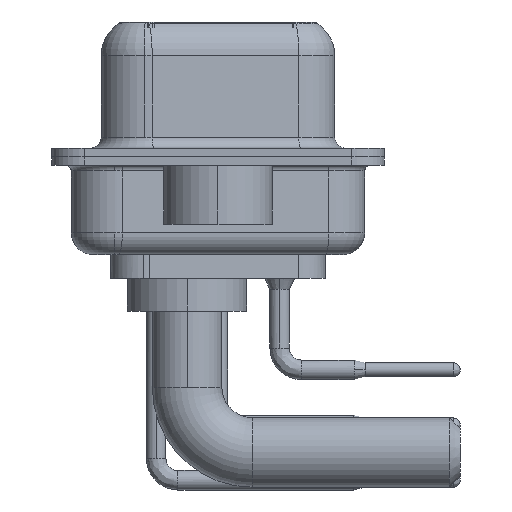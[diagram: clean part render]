
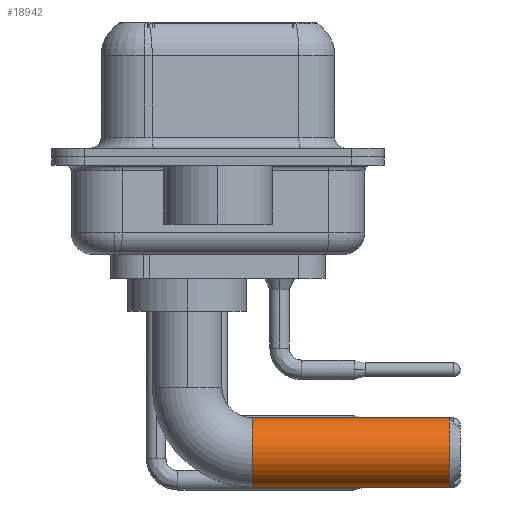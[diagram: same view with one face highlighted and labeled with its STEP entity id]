
A CAD part, left-side view. The second image highlights one B-rep face of the part: STEP entity #18942.
In plain terms, the highlighted cylindrical face has radius 1.6 mm (diameter 3.2 mm), a partial arc.
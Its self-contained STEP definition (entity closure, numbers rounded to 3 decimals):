
#80 = ORIENTED_EDGE ( 'NONE', *, *, #27040, .F. ) ;
#164 = LINE ( 'NONE', #33647, #22647 ) ;
#315 = DIRECTION ( 'NONE',  ( 0., 0., -1. ) ) ;
#1318 = VERTEX_POINT ( 'NONE', #9079 ) ;
#1703 = VERTEX_POINT ( 'NONE', #20347 ) ;
#2631 = DIRECTION ( 'NONE',  ( 0., 0., -1. ) ) ;
#4101 = VERTEX_POINT ( 'NONE', #13779 ) ;
#4811 = CYLINDRICAL_SURFACE ( 'NONE', #26990, 1.6 ) ;
#7614 = DIRECTION ( 'NONE',  ( 0., -1., 0. ) ) ;
#9079 = CARTESIAN_POINT ( 'NONE',  ( 0., -12.07, -8.1 ) ) ;
#9101 = AXIS2_PLACEMENT_3D ( 'NONE', #20648, #7614, #28541 ) ;
#9179 = EDGE_CURVE ( 'NONE', #1703, #18232, #23896, .T. ) ;
#10278 = CIRCLE ( 'NONE', #29450, 1.6 ) ;
#10621 = DIRECTION ( 'NONE',  ( 0., -1., 0. ) ) ;
#11472 = EDGE_CURVE ( 'NONE', #1318, #4101, #10278, .T. ) ;
#12559 = VECTOR ( 'NONE', #32329, 1000. ) ;
#13040 = FACE_OUTER_BOUND ( 'NONE', #27842, .T. ) ;
#13459 = CARTESIAN_POINT ( 'NONE',  ( 0., -3., -8.1 ) ) ;
#13779 = CARTESIAN_POINT ( 'NONE',  ( 0., -12.07, -4.9 ) ) ;
#14502 = ORIENTED_EDGE ( 'NONE', *, *, #9179, .T. ) ;
#15779 = CARTESIAN_POINT ( 'NONE',  ( 0., -3., -6.5 ) ) ;
#15791 = ORIENTED_EDGE ( 'NONE', *, *, #31656, .T. ) ;
#16876 = CARTESIAN_POINT ( 'NONE',  ( 0., -3., -4.9 ) ) ;
#18232 = VERTEX_POINT ( 'NONE', #13459 ) ;
#18499 = DIRECTION ( 'NONE',  ( 0., 1., 0. ) ) ;
#18942 = ADVANCED_FACE ( 'NONE', ( #13040 ), #4811, .T. ) ;
#20347 = CARTESIAN_POINT ( 'NONE',  ( 0., -3., -4.9 ) ) ;
#20648 = CARTESIAN_POINT ( 'NONE',  ( 0., -3., -6.5 ) ) ;
#21097 = DIRECTION ( 'NONE',  ( 0., -1., 0. ) ) ;
#22647 = VECTOR ( 'NONE', #21097, 1000. ) ;
#23896 = CIRCLE ( 'NONE', #9101, 1.6 ) ;
#25885 = CARTESIAN_POINT ( 'NONE',  ( 0., -12.07, -6.5 ) ) ;
#26990 = AXIS2_PLACEMENT_3D ( 'NONE', #15779, #10621, #2631 ) ;
#27040 = EDGE_CURVE ( 'NONE', #1703, #4101, #30260, .T. ) ;
#27256 = ORIENTED_EDGE ( 'NONE', *, *, #11472, .T. ) ;
#27842 = EDGE_LOOP ( 'NONE', ( #80, #14502, #15791, #27256 ) ) ;
#28541 = DIRECTION ( 'NONE',  ( -1., 0., 0. ) ) ;
#29450 = AXIS2_PLACEMENT_3D ( 'NONE', #25885, #18499, #315 ) ;
#30260 = LINE ( 'NONE', #16876, #12559 ) ;
#31656 = EDGE_CURVE ( 'NONE', #18232, #1318, #164, .T. ) ;
#32329 = DIRECTION ( 'NONE',  ( 0., -1., 0. ) ) ;
#33647 = CARTESIAN_POINT ( 'NONE',  ( 0., -3., -8.1 ) ) ;
